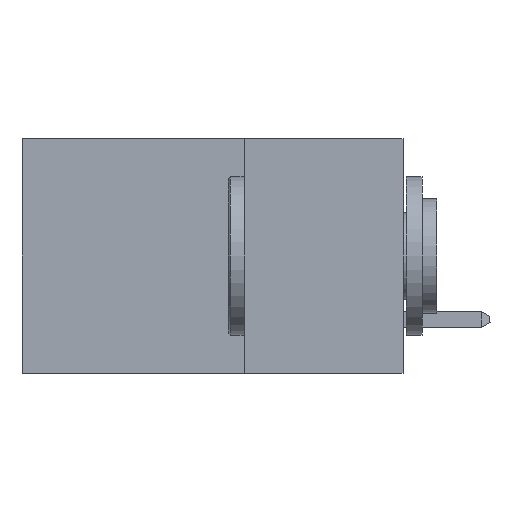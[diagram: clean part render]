
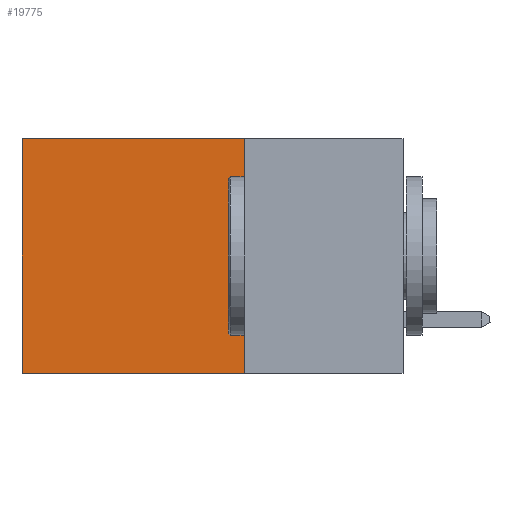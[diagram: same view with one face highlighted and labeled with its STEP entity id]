
A CAD part, left-side view. The second image highlights one B-rep face of the part: STEP entity #19775.
In plain terms, the highlighted planar face has unit normal (-1, 0, 0).
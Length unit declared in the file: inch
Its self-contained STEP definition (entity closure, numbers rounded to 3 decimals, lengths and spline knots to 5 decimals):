
#66 = CARTESIAN_POINT ( 'NONE',  ( 0.2875, 0.6, 0. ) ) ;
#644 = PLANE ( 'NONE',  #33248 ) ;
#916 = FACE_OUTER_BOUND ( 'NONE', #33362, .T. ) ;
#2115 = VERTEX_POINT ( 'NONE', #16693 ) ;
#7254 = DIRECTION ( 'NONE',  ( 0., 1., 0. ) ) ;
#7502 = LINE ( 'NONE', #22042, #36616 ) ;
#9396 = VECTOR ( 'NONE', #21670, 39.37008 ) ;
#10060 = VECTOR ( 'NONE', #32807, 39.37008 ) ;
#11213 = LINE ( 'NONE', #24200, #17831 ) ;
#11821 = DIRECTION ( 'NONE',  ( 0., 0., -1. ) ) ;
#11951 = DIRECTION ( 'NONE',  ( 1., 0., 0. ) ) ;
#14485 = LINE ( 'NONE', #27166, #10060 ) ;
#14805 = CARTESIAN_POINT ( 'NONE',  ( 0.2875, 0.25, 0. ) ) ;
#14978 = ORIENTED_EDGE ( 'NONE', *, *, #19693, .F. ) ;
#16693 = CARTESIAN_POINT ( 'NONE',  ( 0.2875, 0.6, -0.37 ) ) ;
#16953 = LINE ( 'NONE', #18941, #9396 ) ;
#17231 = ORIENTED_EDGE ( 'NONE', *, *, #35852, .F. ) ;
#17831 = VECTOR ( 'NONE', #7254, 39.37008 ) ;
#18722 = ORIENTED_EDGE ( 'NONE', *, *, #35304, .T. ) ;
#18875 = VERTEX_POINT ( 'NONE', #31573 ) ;
#18941 = CARTESIAN_POINT ( 'NONE',  ( 0.2875, 0.25, -0.37 ) ) ;
#19693 = EDGE_CURVE ( 'NONE', #18875, #2115, #16953, .T. ) ;
#19775 = ADVANCED_FACE ( 'NONE', ( #916 ), #644, .F. ) ;
#21670 = DIRECTION ( 'NONE',  ( 0., 1., 0. ) ) ;
#22042 = CARTESIAN_POINT ( 'NONE',  ( 0.2875, 0.6, 0. ) ) ;
#24103 = ORIENTED_EDGE ( 'NONE', *, *, #32339, .T. ) ;
#24200 = CARTESIAN_POINT ( 'NONE',  ( 0.2875, 0.25, 0. ) ) ;
#27166 = CARTESIAN_POINT ( 'NONE',  ( 0.2875, 0.25, 0. ) ) ;
#27711 = DIRECTION ( 'NONE',  ( 0., 0., -1. ) ) ;
#30327 = VERTEX_POINT ( 'NONE', #66 ) ;
#31573 = CARTESIAN_POINT ( 'NONE',  ( 0.2875, 0.25, -0.37 ) ) ;
#32339 = EDGE_CURVE ( 'NONE', #32570, #30327, #11213, .T. ) ;
#32570 = VERTEX_POINT ( 'NONE', #35913 ) ;
#32807 = DIRECTION ( 'NONE',  ( 0., 0., -1. ) ) ;
#33248 = AXIS2_PLACEMENT_3D ( 'NONE', #14805, #11951, #11821 ) ;
#33362 = EDGE_LOOP ( 'NONE', ( #18722, #14978, #17231, #24103 ) ) ;
#35304 = EDGE_CURVE ( 'NONE', #30327, #2115, #7502, .T. ) ;
#35852 = EDGE_CURVE ( 'NONE', #32570, #18875, #14485, .T. ) ;
#35913 = CARTESIAN_POINT ( 'NONE',  ( 0.2875, 0.25, 0. ) ) ;
#36616 = VECTOR ( 'NONE', #27711, 39.37008 ) ;
